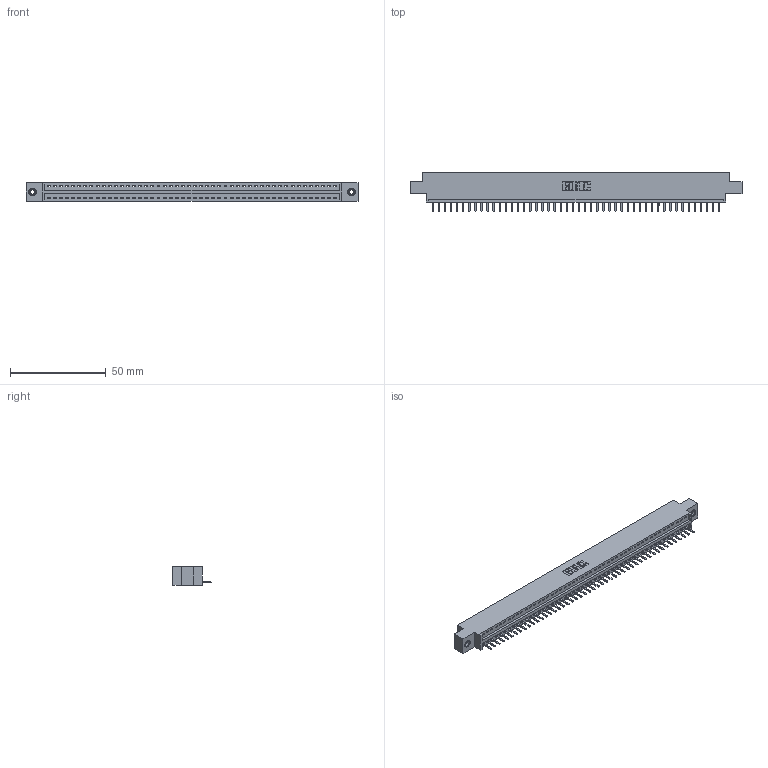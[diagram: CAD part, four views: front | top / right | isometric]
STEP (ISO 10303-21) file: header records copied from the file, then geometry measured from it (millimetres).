
FILE_DESCRIPTION (( 'STEP AP203' ), '1' );
FILE_NAME ('396-048-520-608.STEP', '2018-09-07T11:46:23', ( '' ), ( '' ), 'SwSTEP 2.0', 'SolidWorks 2016', '' );
FILE_SCHEMA (( 'CONFIG_CONTROL_DESIGN' ));
Length unit declared in the file: inch
Products named in the file (4): 396-048-520-608; 346 Part_0.170 Offset - 0.156 Dia-TI; 345-292-001_345-293-120; 345-250-001_345-250-003-102
Assembly tree (51 placements, depth 2):
  396-048-520-608
    346 Part_0.170 Offset - 0.156 Dia-TI
    345-292-001_345-293-120  x48
    345-250-001_345-250-003-102  x2
Bounding box: 172.97 x 20.02 x 9.4 mm (x, y, z)
Volume: 16299.6 mm3; surface area: 20158.3 mm2
Topology: 51 solids, 51 shells, 3162 faces, 9309 edges, 6070 vertices
Faces by surface type: plane 2128, cylinder 1018, cone 12, torus 4
Entity records: 30414 total; most frequent: CARTESIAN_POINT 5207, ORIENTED_EDGE 5170, DIRECTION 4599, EDGE_CURVE 2585, VECTOR 2237, LINE 2237, VERTEX_POINT 1716, AXIS2_PLACEMENT_3D 1181
